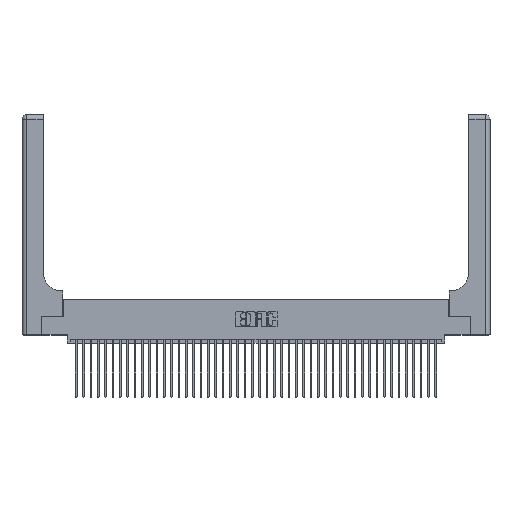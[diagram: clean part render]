
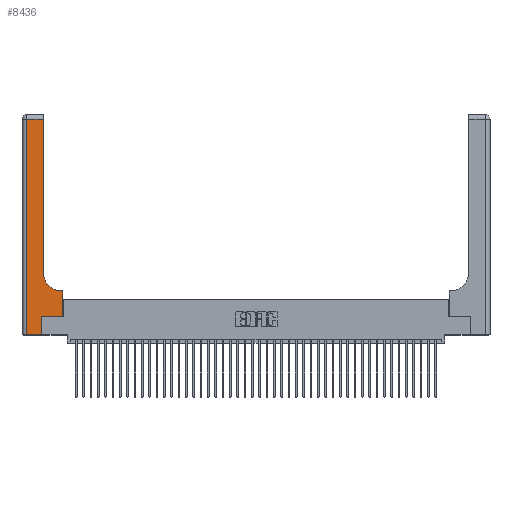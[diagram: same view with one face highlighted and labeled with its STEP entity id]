
A CAD part, top view. The second image highlights one B-rep face of the part: STEP entity #8436.
In plain terms, the highlighted planar face has unit normal (0, 0, 1).
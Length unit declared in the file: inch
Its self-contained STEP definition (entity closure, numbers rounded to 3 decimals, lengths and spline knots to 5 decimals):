
#443 = VECTOR ( 'NONE', #21456, 39.37008 ) ;
#1110 = VECTOR ( 'NONE', #42510, 39.37008 ) ;
#2216 = DIRECTION ( 'NONE',  ( 0., 1., 0. ) ) ;
#2270 = DIRECTION ( 'NONE',  ( 0., 1., 0. ) ) ;
#3055 = CARTESIAN_POINT ( 'NONE',  ( 0.269, 0.25, 0.37 ) ) ;
#3081 = LINE ( 'NONE', #25881, #4127 ) ;
#3101 = VERTEX_POINT ( 'NONE', #3473 ) ;
#3386 = DIRECTION ( 'NONE',  ( 0., 0., -1. ) ) ;
#3473 = CARTESIAN_POINT ( 'NONE',  ( 0.5585, 0.6, 0.37 ) ) ;
#3556 = LINE ( 'NONE', #22473, #4603 ) ;
#3771 = PLANE ( 'NONE',  #36874 ) ;
#4127 = VECTOR ( 'NONE', #2270, 39.37008 ) ;
#4603 = VECTOR ( 'NONE', #2216, 39.37008 ) ;
#4713 = VERTEX_POINT ( 'NONE', #3055 ) ;
#5247 = EDGE_CURVE ( 'NONE', #3101, #15989, #10132, .T. ) ;
#6492 = CARTESIAN_POINT ( 'NONE',  ( 0.5415, 0.85, 0.37 ) ) ;
#6657 = CARTESIAN_POINT ( 'NONE',  ( 0., 3., 0.37 ) ) ;
#6823 = EDGE_CURVE ( 'NONE', #10211, #35299, #13685, .T. ) ;
#8436 = ADVANCED_FACE ( 'NONE', ( #15978 ), #3771, .F. ) ;
#8625 = LINE ( 'NONE', #16082, #16576 ) ;
#9450 = LINE ( 'NONE', #14671, #443 ) ;
#9525 = ORIENTED_EDGE ( 'NONE', *, *, #5247, .T. ) ;
#9886 = DIRECTION ( 'NONE',  ( 1., 0., 0. ) ) ;
#10132 = LINE ( 'NONE', #39154, #1110 ) ;
#10211 = VERTEX_POINT ( 'NONE', #23568 ) ;
#10583 = EDGE_CURVE ( 'NONE', #20593, #3101, #3081, .T. ) ;
#11194 = CARTESIAN_POINT ( 'NONE',  ( 0.06, 3., 0.37 ) ) ;
#11286 = EDGE_CURVE ( 'NONE', #24168, #4713, #3556, .T. ) ;
#12050 = ORIENTED_EDGE ( 'NONE', *, *, #6823, .T. ) ;
#13522 = CARTESIAN_POINT ( 'NONE',  ( 0.2915, 2.94, 0.37 ) ) ;
#13685 = LINE ( 'NONE', #15039, #21612 ) ;
#14455 = CARTESIAN_POINT ( 'NONE',  ( 0.5585, 0.25, 0.37 ) ) ;
#14600 = DIRECTION ( 'NONE',  ( 0., -1., 0. ) ) ;
#14671 = CARTESIAN_POINT ( 'NONE',  ( 0.269, 0.25, 0.37 ) ) ;
#15039 = CARTESIAN_POINT ( 'NONE',  ( 0.2915, 3., 0.37 ) ) ;
#15839 = LINE ( 'NONE', #11194, #42552 ) ;
#15978 = FACE_OUTER_BOUND ( 'NONE', #41807, .T. ) ;
#15989 = VERTEX_POINT ( 'NONE', #19315 ) ;
#16082 = CARTESIAN_POINT ( 'NONE',  ( 0., 0., 0.37 ) ) ;
#16576 = VECTOR ( 'NONE', #42871, 39.37008 ) ;
#16695 = CARTESIAN_POINT ( 'NONE',  ( 0.269, 0., 0.37 ) ) ;
#17632 = EDGE_CURVE ( 'NONE', #35299, #41394, #24833, .T. ) ;
#18806 = EDGE_CURVE ( 'NONE', #41394, #25393, #15839, .T. ) ;
#19315 = CARTESIAN_POINT ( 'NONE',  ( 0.5415, 0.6, 0.37 ) ) ;
#19850 = ORIENTED_EDGE ( 'NONE', *, *, #28224, .T. ) ;
#20593 = VERTEX_POINT ( 'NONE', #14455 ) ;
#21456 = DIRECTION ( 'NONE',  ( 1., 0., 0. ) ) ;
#21612 = VECTOR ( 'NONE', #38468, 39.37008 ) ;
#22473 = CARTESIAN_POINT ( 'NONE',  ( 0.269, 0., 0.37 ) ) ;
#23142 = ORIENTED_EDGE ( 'NONE', *, *, #11286, .T. ) ;
#23568 = CARTESIAN_POINT ( 'NONE',  ( 0.2915, 0.85, 0.37 ) ) ;
#23746 = EDGE_CURVE ( 'NONE', #4713, #20593, #9450, .T. ) ;
#24168 = VERTEX_POINT ( 'NONE', #16695 ) ;
#24833 = LINE ( 'NONE', #30308, #41556 ) ;
#25393 = VERTEX_POINT ( 'NONE', #35623 ) ;
#25728 = CARTESIAN_POINT ( 'NONE',  ( 0.06, 2.94, 0.37 ) ) ;
#25881 = CARTESIAN_POINT ( 'NONE',  ( 0.5585, 0.25, 0.37 ) ) ;
#26477 = AXIS2_PLACEMENT_3D ( 'NONE', #6492, #30023, #9886 ) ;
#26976 = DIRECTION ( 'NONE',  ( -1., 0., 0. ) ) ;
#28224 = EDGE_CURVE ( 'NONE', #25393, #24168, #8625, .T. ) ;
#28290 = EDGE_CURVE ( 'NONE', #15989, #10211, #31258, .T. ) ;
#29821 = ORIENTED_EDGE ( 'NONE', *, *, #10583, .T. ) ;
#30023 = DIRECTION ( 'NONE',  ( 0., 0., -1. ) ) ;
#30308 = CARTESIAN_POINT ( 'NONE',  ( 0., 2.94, 0.37 ) ) ;
#31258 = CIRCLE ( 'NONE', #26477, 0.25 ) ;
#31925 = ORIENTED_EDGE ( 'NONE', *, *, #23746, .T. ) ;
#33689 = DIRECTION ( 'NONE',  ( -1., 0., 0. ) ) ;
#34219 = ORIENTED_EDGE ( 'NONE', *, *, #17632, .T. ) ;
#35299 = VERTEX_POINT ( 'NONE', #13522 ) ;
#35623 = CARTESIAN_POINT ( 'NONE',  ( 0.06, 0., 0.37 ) ) ;
#35721 = ORIENTED_EDGE ( 'NONE', *, *, #28290, .T. ) ;
#36874 = AXIS2_PLACEMENT_3D ( 'NONE', #6657, #3386, #26976 ) ;
#38468 = DIRECTION ( 'NONE',  ( 0., 1., 0. ) ) ;
#39154 = CARTESIAN_POINT ( 'NONE',  ( 0.2915, 0.6, 0.37 ) ) ;
#40784 = ORIENTED_EDGE ( 'NONE', *, *, #18806, .T. ) ;
#41394 = VERTEX_POINT ( 'NONE', #25728 ) ;
#41556 = VECTOR ( 'NONE', #33689, 39.37008 ) ;
#41807 = EDGE_LOOP ( 'NONE', ( #12050, #34219, #40784, #19850, #23142, #31925, #29821, #9525, #35721 ) ) ;
#42510 = DIRECTION ( 'NONE',  ( -1., 0., 0. ) ) ;
#42552 = VECTOR ( 'NONE', #14600, 39.37008 ) ;
#42871 = DIRECTION ( 'NONE',  ( 1., 0., 0. ) ) ;
